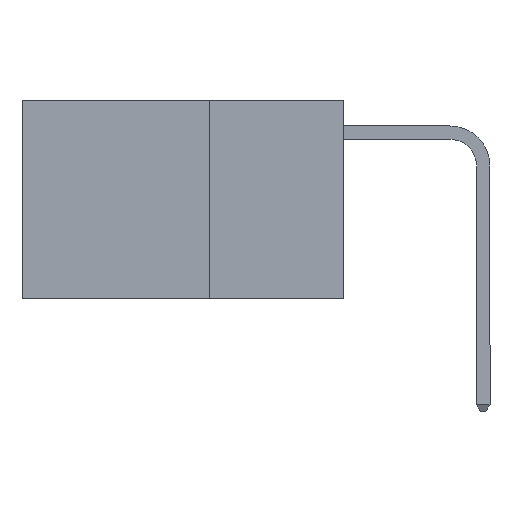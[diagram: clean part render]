
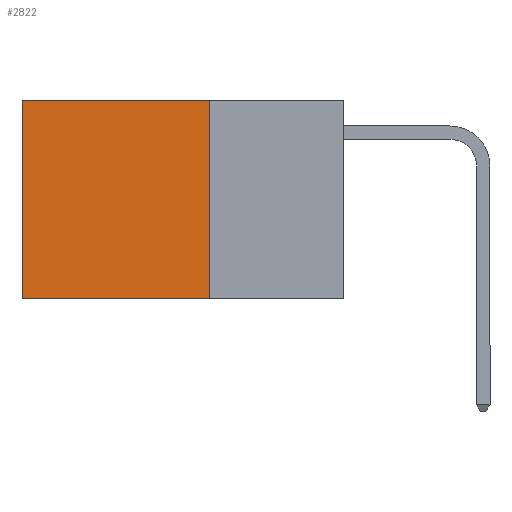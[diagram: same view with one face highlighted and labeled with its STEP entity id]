
A CAD part, left-side view. The second image highlights one B-rep face of the part: STEP entity #2822.
In plain terms, the highlighted planar face has unit normal (-1, 0, 0).
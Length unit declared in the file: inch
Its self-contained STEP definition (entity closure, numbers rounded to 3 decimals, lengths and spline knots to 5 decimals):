
#83 = VERTEX_POINT ( 'NONE', #7557 ) ;
#146 = EDGE_CURVE ( 'NONE', #9859, #5261, #1509, .T. ) ;
#974 = VECTOR ( 'NONE', #6339, 39.37008 ) ;
#1379 = AXIS2_PLACEMENT_3D ( 'NONE', #3791, #3764, #3746 ) ;
#1508 = CARTESIAN_POINT ( 'NONE',  ( 0.2625, 0.25, -0.37 ) ) ;
#1509 = LINE ( 'NONE', #7128, #8563 ) ;
#2822 = ADVANCED_FACE ( 'NONE', ( #4968 ), #4059, .F. ) ;
#2847 = CARTESIAN_POINT ( 'NONE',  ( 0.2625, 0.25, 0. ) ) ;
#2856 = CARTESIAN_POINT ( 'NONE',  ( 0.2625, 0.6, -0.37 ) ) ;
#3587 = EDGE_LOOP ( 'NONE', ( #9124, #8068, #11562, #5231 ) ) ;
#3746 = DIRECTION ( 'NONE',  ( 0., 0., -1. ) ) ;
#3764 = DIRECTION ( 'NONE',  ( 1., 0., 0. ) ) ;
#3791 = CARTESIAN_POINT ( 'NONE',  ( 0.2625, 0.25, 0. ) ) ;
#3974 = DIRECTION ( 'NONE',  ( 0., 1., 0. ) ) ;
#4059 = PLANE ( 'NONE',  #1379 ) ;
#4221 = LINE ( 'NONE', #7155, #974 ) ;
#4824 = VECTOR ( 'NONE', #3974, 39.37008 ) ;
#4865 = EDGE_CURVE ( 'NONE', #9859, #83, #8973, .T. ) ;
#4968 = FACE_OUTER_BOUND ( 'NONE', #3587, .T. ) ;
#5191 = CARTESIAN_POINT ( 'NONE',  ( 0.2625, 0.25, -0.37 ) ) ;
#5231 = ORIENTED_EDGE ( 'NONE', *, *, #4865, .T. ) ;
#5261 = VERTEX_POINT ( 'NONE', #5191 ) ;
#5779 = VECTOR ( 'NONE', #8839, 39.37008 ) ;
#6339 = DIRECTION ( 'NONE',  ( 0., 0., -1. ) ) ;
#7128 = CARTESIAN_POINT ( 'NONE',  ( 0.2625, 0.25, 0. ) ) ;
#7155 = CARTESIAN_POINT ( 'NONE',  ( 0.2625, 0.6, 0. ) ) ;
#7184 = CARTESIAN_POINT ( 'NONE',  ( 0.2625, 0.25, 0. ) ) ;
#7557 = CARTESIAN_POINT ( 'NONE',  ( 0.2625, 0.6, 0. ) ) ;
#8068 = ORIENTED_EDGE ( 'NONE', *, *, #10957, .F. ) ;
#8563 = VECTOR ( 'NONE', #9012, 39.37008 ) ;
#8839 = DIRECTION ( 'NONE',  ( 0., 1., 0. ) ) ;
#8912 = EDGE_CURVE ( 'NONE', #83, #11299, #4221, .T. ) ;
#8973 = LINE ( 'NONE', #2847, #4824 ) ;
#9012 = DIRECTION ( 'NONE',  ( 0., 0., -1. ) ) ;
#9124 = ORIENTED_EDGE ( 'NONE', *, *, #8912, .T. ) ;
#9859 = VERTEX_POINT ( 'NONE', #7184 ) ;
#10957 = EDGE_CURVE ( 'NONE', #5261, #11299, #11492, .T. ) ;
#11299 = VERTEX_POINT ( 'NONE', #2856 ) ;
#11492 = LINE ( 'NONE', #1508, #5779 ) ;
#11562 = ORIENTED_EDGE ( 'NONE', *, *, #146, .F. ) ;
